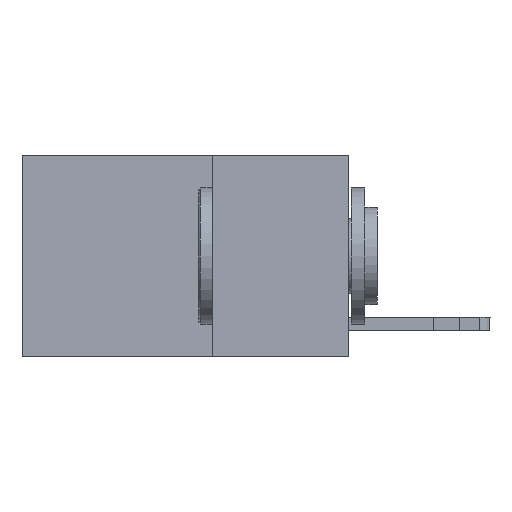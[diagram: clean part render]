
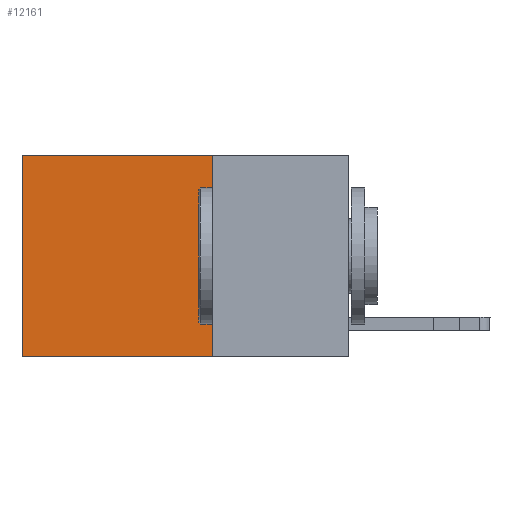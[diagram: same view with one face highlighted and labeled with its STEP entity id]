
A CAD part, left-side view. The second image highlights one B-rep face of the part: STEP entity #12161.
In plain terms, the highlighted planar face has unit normal (-1, 0, 0).
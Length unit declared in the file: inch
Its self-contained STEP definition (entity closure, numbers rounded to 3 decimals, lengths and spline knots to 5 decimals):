
#931 = AXIS2_PLACEMENT_3D ( 'NONE', #7010, #4153, #14528 ) ;
#997 = LINE ( 'NONE', #5022, #13432 ) ;
#1033 = PLANE ( 'NONE',  #931 ) ;
#1582 = EDGE_CURVE ( 'NONE', #6551, #18652, #2480, .T. ) ;
#1811 = EDGE_LOOP ( 'NONE', ( #2124, #3593, #16799, #2784 ) ) ;
#1858 = EDGE_CURVE ( 'NONE', #5983, #13978, #14134, .T. ) ;
#2124 = ORIENTED_EDGE ( 'NONE', *, *, #1582, .T. ) ;
#2349 = CARTESIAN_POINT ( 'NONE',  ( 0.2625, 0.25, -0.37 ) ) ;
#2480 = LINE ( 'NONE', #7046, #17793 ) ;
#2784 = ORIENTED_EDGE ( 'NONE', *, *, #17498, .T. ) ;
#3593 = ORIENTED_EDGE ( 'NONE', *, *, #13169, .F. ) ;
#3777 = CARTESIAN_POINT ( 'NONE',  ( 0.2625, 0.25, 0. ) ) ;
#4153 = DIRECTION ( 'NONE',  ( 1., 0., 0. ) ) ;
#5022 = CARTESIAN_POINT ( 'NONE',  ( 0.2625, 0.25, -0.37 ) ) ;
#5983 = VERTEX_POINT ( 'NONE', #3777 ) ;
#6124 = DIRECTION ( 'NONE',  ( 0., 0., -1. ) ) ;
#6551 = VERTEX_POINT ( 'NONE', #9548 ) ;
#7010 = CARTESIAN_POINT ( 'NONE',  ( 0.2625, 0.25, 0. ) ) ;
#7046 = CARTESIAN_POINT ( 'NONE',  ( 0.2625, 0.6, 0. ) ) ;
#7445 = DIRECTION ( 'NONE',  ( 0., 0., -1. ) ) ;
#8078 = LINE ( 'NONE', #13577, #15463 ) ;
#9548 = CARTESIAN_POINT ( 'NONE',  ( 0.2625, 0.6, 0. ) ) ;
#10008 = FACE_OUTER_BOUND ( 'NONE', #1811, .T. ) ;
#10669 = DIRECTION ( 'NONE',  ( 0., 1., 0. ) ) ;
#11732 = CARTESIAN_POINT ( 'NONE',  ( 0.2625, 0.25, 0. ) ) ;
#12161 = ADVANCED_FACE ( 'NONE', ( #10008 ), #1033, .F. ) ;
#13169 = EDGE_CURVE ( 'NONE', #13978, #18652, #997, .T. ) ;
#13432 = VECTOR ( 'NONE', #15379, 39.37008 ) ;
#13577 = CARTESIAN_POINT ( 'NONE',  ( 0.2625, 0.25, 0. ) ) ;
#13978 = VERTEX_POINT ( 'NONE', #2349 ) ;
#14134 = LINE ( 'NONE', #11732, #18952 ) ;
#14528 = DIRECTION ( 'NONE',  ( 0., 0., -1. ) ) ;
#15379 = DIRECTION ( 'NONE',  ( 0., 1., 0. ) ) ;
#15463 = VECTOR ( 'NONE', #10669, 39.37008 ) ;
#16799 = ORIENTED_EDGE ( 'NONE', *, *, #1858, .F. ) ;
#17498 = EDGE_CURVE ( 'NONE', #5983, #6551, #8078, .T. ) ;
#17793 = VECTOR ( 'NONE', #6124, 39.37008 ) ;
#18652 = VERTEX_POINT ( 'NONE', #18931 ) ;
#18931 = CARTESIAN_POINT ( 'NONE',  ( 0.2625, 0.6, -0.37 ) ) ;
#18952 = VECTOR ( 'NONE', #7445, 39.37008 ) ;
